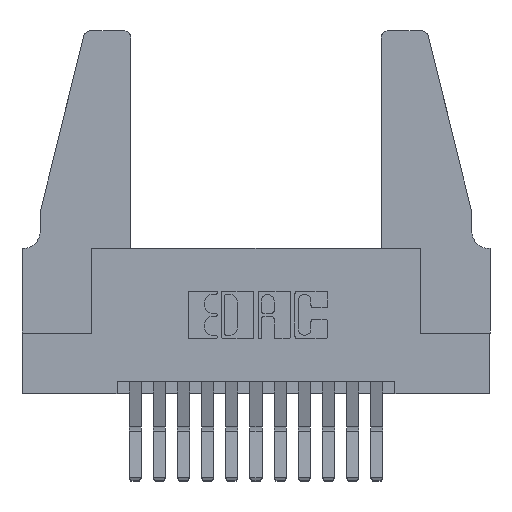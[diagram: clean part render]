
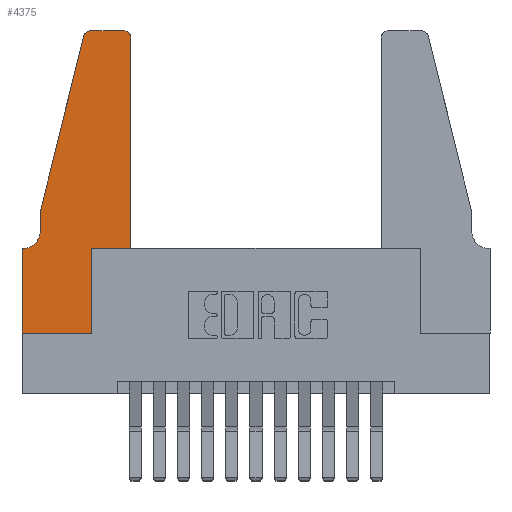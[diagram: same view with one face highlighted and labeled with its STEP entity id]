
A CAD part, top view. The second image highlights one B-rep face of the part: STEP entity #4375.
In plain terms, the highlighted planar face has unit normal (0, 0, 1).
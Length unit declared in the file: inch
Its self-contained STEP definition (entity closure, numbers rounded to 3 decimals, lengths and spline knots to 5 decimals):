
#287 = CIRCLE ( 'NONE', #6378, 0.03 ) ;
#326 = ORIENTED_EDGE ( 'NONE', *, *, #724, .T. ) ;
#482 = DIRECTION ( 'NONE',  ( 0., 1., 0. ) ) ;
#565 = CARTESIAN_POINT ( 'NONE',  ( 0.0755, 0.35, 0.37 ) ) ;
#724 = EDGE_CURVE ( 'NONE', #7841, #2857, #1655, .T. ) ;
#920 = ORIENTED_EDGE ( 'NONE', *, *, #8729, .T. ) ;
#973 = VERTEX_POINT ( 'NONE', #4296 ) ;
#1178 = CARTESIAN_POINT ( 'NONE',  ( 0.4505, 0.35, 0.37 ) ) ;
#1297 = VECTOR ( 'NONE', #14015, 39.37008 ) ;
#1370 = VECTOR ( 'NONE', #8068, 39.37008 ) ;
#1555 = VERTEX_POINT ( 'NONE', #8984 ) ;
#1655 = LINE ( 'NONE', #4391, #1297 ) ;
#1739 = ORIENTED_EDGE ( 'NONE', *, *, #2766, .T. ) ;
#2168 = DIRECTION ( 'NONE',  ( 1., 0., 0. ) ) ;
#2200 = CARTESIAN_POINT ( 'NONE',  ( 0.0755, 0.5, 0.37 ) ) ;
#2307 = EDGE_CURVE ( 'NONE', #13677, #1555, #3481, .T. ) ;
#2331 = VECTOR ( 'NONE', #3622, 39.37008 ) ;
#2351 = ORIENTED_EDGE ( 'NONE', *, *, #8289, .T. ) ;
#2766 = EDGE_CURVE ( 'NONE', #4530, #10344, #4592, .T. ) ;
#2815 = AXIS2_PLACEMENT_3D ( 'NONE', #3826, #12531, #3772 ) ;
#2857 = VERTEX_POINT ( 'NONE', #6390 ) ;
#2862 = CARTESIAN_POINT ( 'NONE',  ( 0., 0.35, 0.37 ) ) ;
#3001 = VECTOR ( 'NONE', #14365, 39.37008 ) ;
#3262 = VERTEX_POINT ( 'NONE', #7960 ) ;
#3404 = CARTESIAN_POINT ( 'NONE',  ( 0.2865, 0.35, 0.37 ) ) ;
#3481 = LINE ( 'NONE', #8708, #13752 ) ;
#3555 = VERTEX_POINT ( 'NONE', #3404 ) ;
#3622 = DIRECTION ( 'NONE',  ( 1., 0., 0. ) ) ;
#3646 = VECTOR ( 'NONE', #13003, 39.37008 ) ;
#3772 = DIRECTION ( 'NONE',  ( -1., 0., 0. ) ) ;
#3826 = CARTESIAN_POINT ( 'NONE',  ( 0.0055, 0.42, 0.37 ) ) ;
#4021 = LINE ( 'NONE', #8505, #3646 ) ;
#4296 = CARTESIAN_POINT ( 'NONE',  ( 0.2865, 0., 0.37 ) ) ;
#4375 = ADVANCED_FACE ( 'NONE', ( #4931 ), #13689, .T. ) ;
#4391 = CARTESIAN_POINT ( 'NONE',  ( 0.0755, 0.5, 0.37 ) ) ;
#4530 = VERTEX_POINT ( 'NONE', #11716 ) ;
#4592 = CIRCLE ( 'NONE', #2815, 0.07 ) ;
#4898 = LINE ( 'NONE', #565, #11016 ) ;
#4931 = FACE_OUTER_BOUND ( 'NONE', #11781, .T. ) ;
#5121 = AXIS2_PLACEMENT_3D ( 'NONE', #5811, #13812, #6981 ) ;
#5185 = CARTESIAN_POINT ( 'NONE',  ( 0.4205, 1.22, 0.37 ) ) ;
#5472 = ORIENTED_EDGE ( 'NONE', *, *, #7213, .T. ) ;
#5476 = LINE ( 'NONE', #8278, #2331 ) ;
#5685 = CARTESIAN_POINT ( 'NONE',  ( 0.4505, 1.22, 0.37 ) ) ;
#5811 = CARTESIAN_POINT ( 'NONE',  ( 0.284, 1.22, 0.37 ) ) ;
#6032 = CARTESIAN_POINT ( 'NONE',  ( 0.284, 1.25, 0.37 ) ) ;
#6342 = DIRECTION ( 'NONE',  ( 1., 0., 0. ) ) ;
#6378 = AXIS2_PLACEMENT_3D ( 'NONE', #5185, #13198, #6342 ) ;
#6390 = CARTESIAN_POINT ( 'NONE',  ( 0.0755, 0.5, 0.37 ) ) ;
#6883 = LINE ( 'NONE', #13201, #3001 ) ;
#6981 = DIRECTION ( 'NONE',  ( 1., 0., 0. ) ) ;
#7088 = ORIENTED_EDGE ( 'NONE', *, *, #9296, .T. ) ;
#7213 = EDGE_CURVE ( 'NONE', #9930, #11110, #4021, .T. ) ;
#7711 = EDGE_CURVE ( 'NONE', #3262, #9577, #11770, .T. ) ;
#7841 = VERTEX_POINT ( 'NONE', #9553 ) ;
#7960 = CARTESIAN_POINT ( 'NONE',  ( 0.4505, 0.35, 0.37 ) ) ;
#8068 = DIRECTION ( 'NONE',  ( 0., -1., 0. ) ) ;
#8278 = CARTESIAN_POINT ( 'NONE',  ( 0., 0., 0.37 ) ) ;
#8289 = EDGE_CURVE ( 'NONE', #2857, #4530, #13687, .T. ) ;
#8505 = CARTESIAN_POINT ( 'NONE',  ( 0.2605, 1.25, 0.37 ) ) ;
#8677 = DIRECTION ( 'NONE',  ( 0., -1., 0. ) ) ;
#8708 = CARTESIAN_POINT ( 'NONE',  ( 0., 0., 0.37 ) ) ;
#8729 = EDGE_CURVE ( 'NONE', #10344, #13677, #4898, .T. ) ;
#8861 = DIRECTION ( 'NONE',  ( -1., 0., 0. ) ) ;
#8984 = CARTESIAN_POINT ( 'NONE',  ( 0., 0., 0.37 ) ) ;
#9210 = DIRECTION ( 'NONE',  ( 0., 0., 1. ) ) ;
#9228 = AXIS2_PLACEMENT_3D ( 'NONE', #13639, #9210, #2168 ) ;
#9296 = EDGE_CURVE ( 'NONE', #3555, #3262, #6883, .T. ) ;
#9405 = DIRECTION ( 'NONE',  ( 0., 1., 0. ) ) ;
#9444 = ORIENTED_EDGE ( 'NONE', *, *, #13984, .T. ) ;
#9513 = ORIENTED_EDGE ( 'NONE', *, *, #14725, .T. ) ;
#9515 = LINE ( 'NONE', #9830, #12142 ) ;
#9553 = CARTESIAN_POINT ( 'NONE',  ( 0.25487, 1.22718, 0.37 ) ) ;
#9577 = VERTEX_POINT ( 'NONE', #5685 ) ;
#9830 = CARTESIAN_POINT ( 'NONE',  ( 0.2865, 0.35, 0.37 ) ) ;
#9930 = VERTEX_POINT ( 'NONE', #10837 ) ;
#10344 = VERTEX_POINT ( 'NONE', #10436 ) ;
#10436 = CARTESIAN_POINT ( 'NONE',  ( 0.0055, 0.35, 0.37 ) ) ;
#10837 = CARTESIAN_POINT ( 'NONE',  ( 0.4205, 1.25, 0.37 ) ) ;
#11016 = VECTOR ( 'NONE', #8861, 39.37008 ) ;
#11110 = VERTEX_POINT ( 'NONE', #6032 ) ;
#11716 = CARTESIAN_POINT ( 'NONE',  ( 0.0755, 0.42, 0.37 ) ) ;
#11770 = LINE ( 'NONE', #1178, #12457 ) ;
#11781 = EDGE_LOOP ( 'NONE', ( #5472, #9444, #326, #2351, #1739, #920, #12713, #9513, #12414, #7088, #13309, #12703 ) ) ;
#12142 = VECTOR ( 'NONE', #482, 39.37008 ) ;
#12144 = CIRCLE ( 'NONE', #5121, 0.03 ) ;
#12414 = ORIENTED_EDGE ( 'NONE', *, *, #13011, .T. ) ;
#12457 = VECTOR ( 'NONE', #9405, 39.37008 ) ;
#12531 = DIRECTION ( 'NONE',  ( 0., 0., -1. ) ) ;
#12703 = ORIENTED_EDGE ( 'NONE', *, *, #14305, .T. ) ;
#12713 = ORIENTED_EDGE ( 'NONE', *, *, #2307, .T. ) ;
#13003 = DIRECTION ( 'NONE',  ( -1., 0., 0. ) ) ;
#13011 = EDGE_CURVE ( 'NONE', #973, #3555, #9515, .T. ) ;
#13198 = DIRECTION ( 'NONE',  ( 0., 0., 1. ) ) ;
#13201 = CARTESIAN_POINT ( 'NONE',  ( 0.4505, 0.35, 0.37 ) ) ;
#13309 = ORIENTED_EDGE ( 'NONE', *, *, #7711, .T. ) ;
#13639 = CARTESIAN_POINT ( 'NONE',  ( 0., 0.35, 0.37 ) ) ;
#13677 = VERTEX_POINT ( 'NONE', #2862 ) ;
#13687 = LINE ( 'NONE', #2200, #1370 ) ;
#13689 = PLANE ( 'NONE',  #9228 ) ;
#13752 = VECTOR ( 'NONE', #8677, 39.37008 ) ;
#13812 = DIRECTION ( 'NONE',  ( 0., 0., 1. ) ) ;
#13984 = EDGE_CURVE ( 'NONE', #11110, #7841, #12144, .T. ) ;
#14015 = DIRECTION ( 'NONE',  ( -0.239, -0.971, 0. ) ) ;
#14305 = EDGE_CURVE ( 'NONE', #9577, #9930, #287, .T. ) ;
#14365 = DIRECTION ( 'NONE',  ( 1., 0., 0. ) ) ;
#14725 = EDGE_CURVE ( 'NONE', #1555, #973, #5476, .T. ) ;
